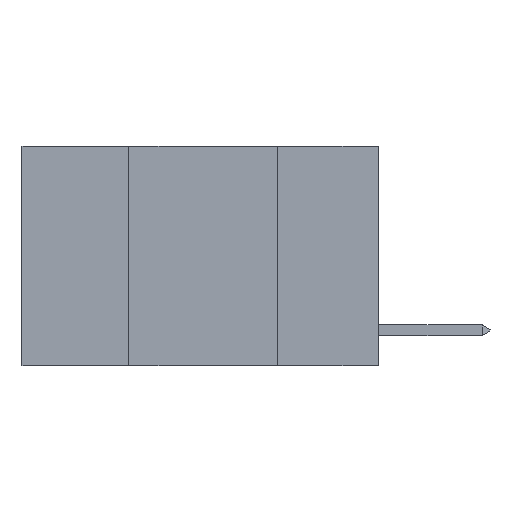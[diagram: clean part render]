
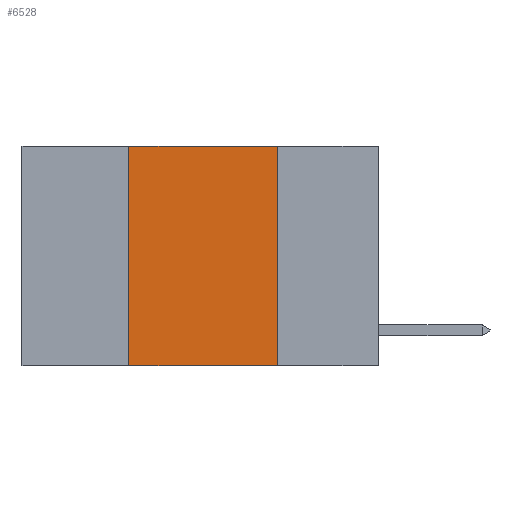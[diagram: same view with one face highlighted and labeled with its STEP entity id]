
A CAD part, left-side view. The second image highlights one B-rep face of the part: STEP entity #6528.
In plain terms, the highlighted planar face has unit normal (-1, 0, 0).
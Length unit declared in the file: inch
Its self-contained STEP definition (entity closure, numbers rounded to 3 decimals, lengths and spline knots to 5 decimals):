
#179 = FACE_OUTER_BOUND ( 'NONE', #6272, .T. ) ;
#538 = VERTEX_POINT ( 'NONE', #1964 ) ;
#701 = AXIS2_PLACEMENT_3D ( 'NONE', #3452, #7696, #6350 ) ;
#1964 = CARTESIAN_POINT ( 'NONE',  ( 0., 0.42, 0. ) ) ;
#2107 = LINE ( 'NONE', #6367, #11823 ) ;
#2301 = VERTEX_POINT ( 'NONE', #9712 ) ;
#3031 = ORIENTED_EDGE ( 'NONE', *, *, #12146, .F. ) ;
#3452 = CARTESIAN_POINT ( 'NONE',  ( 0., 0.6, 0. ) ) ;
#5384 = VECTOR ( 'NONE', #7071, 39.37008 ) ;
#5985 = EDGE_CURVE ( 'NONE', #2301, #9475, #2107, .T. ) ;
#6058 = LINE ( 'NONE', #10356, #10274 ) ;
#6204 = LINE ( 'NONE', #13699, #5384 ) ;
#6214 = VECTOR ( 'NONE', #8167, 39.37008 ) ;
#6272 = EDGE_LOOP ( 'NONE', ( #3031, #13217, #9320, #10377 ) ) ;
#6350 = DIRECTION ( 'NONE',  ( 0., 0., -1. ) ) ;
#6367 = CARTESIAN_POINT ( 'NONE',  ( 0., 0.6, -0.37 ) ) ;
#6528 = ADVANCED_FACE ( 'NONE', ( #179 ), #13042, .F. ) ;
#7071 = DIRECTION ( 'NONE',  ( 0., 0., 1. ) ) ;
#7110 = CARTESIAN_POINT ( 'NONE',  ( 0., 0.17, 0. ) ) ;
#7696 = DIRECTION ( 'NONE',  ( 1., 0., 0. ) ) ;
#8167 = DIRECTION ( 'NONE',  ( 0., -1., 0. ) ) ;
#8676 = CARTESIAN_POINT ( 'NONE',  ( 0., 0.17, -0.37 ) ) ;
#8874 = EDGE_CURVE ( 'NONE', #538, #12615, #9336, .T. ) ;
#9320 = ORIENTED_EDGE ( 'NONE', *, *, #9707, .F. ) ;
#9336 = LINE ( 'NONE', #11555, #6214 ) ;
#9475 = VERTEX_POINT ( 'NONE', #8676 ) ;
#9707 = EDGE_CURVE ( 'NONE', #2301, #538, #6204, .T. ) ;
#9712 = CARTESIAN_POINT ( 'NONE',  ( 0., 0.42, -0.37 ) ) ;
#10205 = DIRECTION ( 'NONE',  ( 0., 0., -1. ) ) ;
#10274 = VECTOR ( 'NONE', #10205, 39.37008 ) ;
#10356 = CARTESIAN_POINT ( 'NONE',  ( 0., 0.17, 0. ) ) ;
#10377 = ORIENTED_EDGE ( 'NONE', *, *, #5985, .T. ) ;
#10622 = DIRECTION ( 'NONE',  ( 0., -1., 0. ) ) ;
#11555 = CARTESIAN_POINT ( 'NONE',  ( 0., 0.6, 0. ) ) ;
#11823 = VECTOR ( 'NONE', #10622, 39.37008 ) ;
#12146 = EDGE_CURVE ( 'NONE', #12615, #9475, #6058, .T. ) ;
#12615 = VERTEX_POINT ( 'NONE', #7110 ) ;
#13042 = PLANE ( 'NONE',  #701 ) ;
#13217 = ORIENTED_EDGE ( 'NONE', *, *, #8874, .F. ) ;
#13699 = CARTESIAN_POINT ( 'NONE',  ( 0., 0.42, 0. ) ) ;
